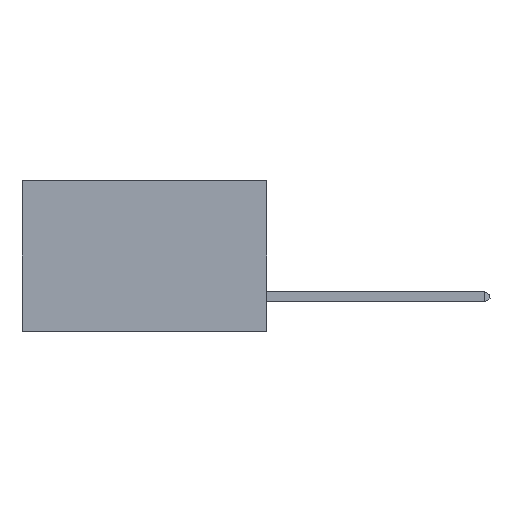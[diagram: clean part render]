
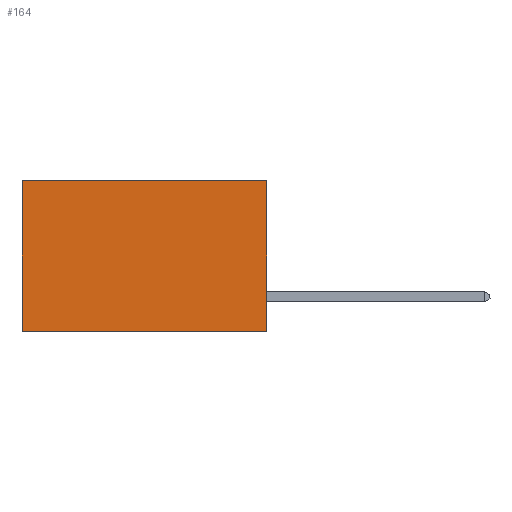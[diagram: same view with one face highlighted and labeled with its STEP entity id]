
A CAD part, left-side view. The second image highlights one B-rep face of the part: STEP entity #164.
In plain terms, the highlighted planar face has unit normal (-1, 0, 0).
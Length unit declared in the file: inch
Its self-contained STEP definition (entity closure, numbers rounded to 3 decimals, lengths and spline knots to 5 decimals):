
#164 = ADVANCED_FACE ( 'NONE', ( #8645 ), #989, .F. ) ;
#258 = LINE ( 'NONE', #10493, #9107 ) ;
#334 = VECTOR ( 'NONE', #1680, 39.37008 ) ;
#604 = AXIS2_PLACEMENT_3D ( 'NONE', #1953, #7769, #2842 ) ;
#989 = PLANE ( 'NONE',  #604 ) ;
#1680 = DIRECTION ( 'NONE',  ( 0., 1., 0. ) ) ;
#1795 = CARTESIAN_POINT ( 'NONE',  ( 0.2875, 0., 0. ) ) ;
#1888 = CARTESIAN_POINT ( 'NONE',  ( 0.2875, 0., -0.37 ) ) ;
#1953 = CARTESIAN_POINT ( 'NONE',  ( 0.2875, 0., 0. ) ) ;
#2092 = CARTESIAN_POINT ( 'NONE',  ( 0.2875, 0., 0. ) ) ;
#2108 = ORIENTED_EDGE ( 'NONE', *, *, #4653, .T. ) ;
#2247 = ORIENTED_EDGE ( 'NONE', *, *, #7438, .F. ) ;
#2274 = EDGE_LOOP ( 'NONE', ( #2108, #7052, #2247, #10787 ) ) ;
#2842 = DIRECTION ( 'NONE',  ( 0., 0., -1. ) ) ;
#3250 = VECTOR ( 'NONE', #10479, 39.37008 ) ;
#3506 = CARTESIAN_POINT ( 'NONE',  ( 0.2875, 0.6, -0.37 ) ) ;
#3523 = LINE ( 'NONE', #10561, #3250 ) ;
#4241 = CARTESIAN_POINT ( 'NONE',  ( 0.2875, 0.6, 0. ) ) ;
#4653 = EDGE_CURVE ( 'NONE', #7692, #8113, #10634, .T. ) ;
#5300 = EDGE_CURVE ( 'NONE', #6447, #7692, #9148, .T. ) ;
#5929 = EDGE_CURVE ( 'NONE', #7566, #8113, #3523, .T. ) ;
#6375 = VECTOR ( 'NONE', #9066, 39.37008 ) ;
#6447 = VERTEX_POINT ( 'NONE', #2092 ) ;
#7052 = ORIENTED_EDGE ( 'NONE', *, *, #5929, .F. ) ;
#7438 = EDGE_CURVE ( 'NONE', #6447, #7566, #258, .T. ) ;
#7566 = VERTEX_POINT ( 'NONE', #1888 ) ;
#7692 = VERTEX_POINT ( 'NONE', #4241 ) ;
#7743 = DIRECTION ( 'NONE',  ( 0., 0., -1. ) ) ;
#7769 = DIRECTION ( 'NONE',  ( 1., 0., 0. ) ) ;
#8113 = VERTEX_POINT ( 'NONE', #3506 ) ;
#8645 = FACE_OUTER_BOUND ( 'NONE', #2274, .T. ) ;
#9066 = DIRECTION ( 'NONE',  ( 0., 0., -1. ) ) ;
#9107 = VECTOR ( 'NONE', #7743, 39.37008 ) ;
#9120 = CARTESIAN_POINT ( 'NONE',  ( 0.2875, 0.6, 0. ) ) ;
#9148 = LINE ( 'NONE', #1795, #334 ) ;
#10479 = DIRECTION ( 'NONE',  ( 0., 1., 0. ) ) ;
#10493 = CARTESIAN_POINT ( 'NONE',  ( 0.2875, 0., 0. ) ) ;
#10561 = CARTESIAN_POINT ( 'NONE',  ( 0.2875, 0., -0.37 ) ) ;
#10634 = LINE ( 'NONE', #9120, #6375 ) ;
#10787 = ORIENTED_EDGE ( 'NONE', *, *, #5300, .T. ) ;
